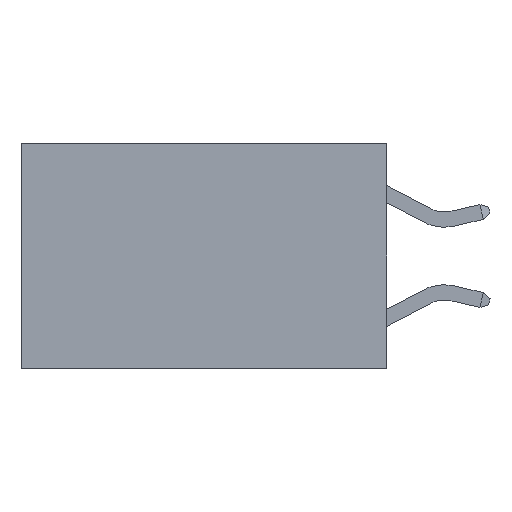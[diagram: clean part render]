
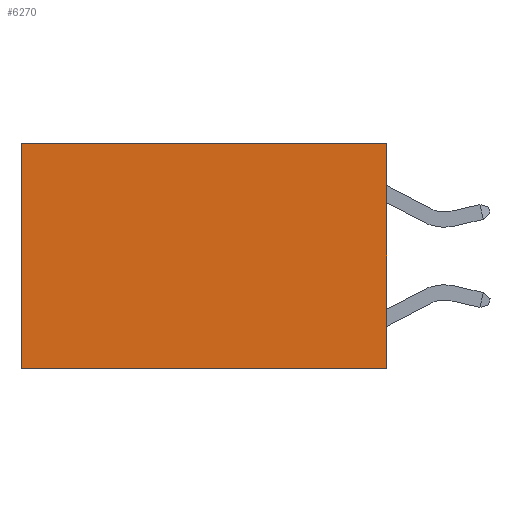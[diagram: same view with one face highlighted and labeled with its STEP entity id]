
A CAD part, left-side view. The second image highlights one B-rep face of the part: STEP entity #6270.
In plain terms, the highlighted planar face has unit normal (-1, 0, 0).
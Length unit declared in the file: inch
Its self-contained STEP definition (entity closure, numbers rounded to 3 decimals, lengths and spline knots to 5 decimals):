
#98 = ORIENTED_EDGE ( 'NONE', *, *, #858, .T. ) ;
#239 = VERTEX_POINT ( 'NONE', #744 ) ;
#382 = ORIENTED_EDGE ( 'NONE', *, *, #1693, .F. ) ;
#744 = CARTESIAN_POINT ( 'NONE',  ( 0.2625, 0.6, -0.37 ) ) ;
#858 = EDGE_CURVE ( 'NONE', #6455, #4580, #6442, .T. ) ;
#1083 = VERTEX_POINT ( 'NONE', #4020 ) ;
#1142 = EDGE_CURVE ( 'NONE', #6455, #1083, #1445, .T. ) ;
#1215 = AXIS2_PLACEMENT_3D ( 'NONE', #2213, #2033, #2023 ) ;
#1445 = LINE ( 'NONE', #8129, #4918 ) ;
#1579 = ORIENTED_EDGE ( 'NONE', *, *, #7103, .T. ) ;
#1693 = EDGE_CURVE ( 'NONE', #1083, #239, #5097, .T. ) ;
#2023 = DIRECTION ( 'NONE',  ( 0., 0., -1. ) ) ;
#2033 = DIRECTION ( 'NONE',  ( 1., 0., 0. ) ) ;
#2051 = PLANE ( 'NONE',  #1215 ) ;
#2061 = CARTESIAN_POINT ( 'NONE',  ( 0.2625, 0.6, 0. ) ) ;
#2064 = VECTOR ( 'NONE', #5233, 39.37008 ) ;
#2213 = CARTESIAN_POINT ( 'NONE',  ( 0.2625, 0., 0. ) ) ;
#3432 = DIRECTION ( 'NONE',  ( 0., 1., 0. ) ) ;
#3454 = EDGE_LOOP ( 'NONE', ( #1579, #382, #8194, #98 ) ) ;
#3459 = CARTESIAN_POINT ( 'NONE',  ( 0.2625, 0., -0.37 ) ) ;
#4020 = CARTESIAN_POINT ( 'NONE',  ( 0.2625, 0., -0.37 ) ) ;
#4046 = LINE ( 'NONE', #7254, #2064 ) ;
#4580 = VERTEX_POINT ( 'NONE', #2061 ) ;
#4609 = DIRECTION ( 'NONE',  ( 0., 0., -1. ) ) ;
#4611 = VECTOR ( 'NONE', #7429, 39.37008 ) ;
#4701 = VECTOR ( 'NONE', #3432, 39.37008 ) ;
#4918 = VECTOR ( 'NONE', #4609, 39.37008 ) ;
#5097 = LINE ( 'NONE', #3459, #4701 ) ;
#5233 = DIRECTION ( 'NONE',  ( 0., 0., -1. ) ) ;
#5687 = CARTESIAN_POINT ( 'NONE',  ( 0.2625, 0., 0. ) ) ;
#5986 = FACE_OUTER_BOUND ( 'NONE', #3454, .T. ) ;
#6270 = ADVANCED_FACE ( 'NONE', ( #5986 ), #2051, .F. ) ;
#6442 = LINE ( 'NONE', #7573, #4611 ) ;
#6455 = VERTEX_POINT ( 'NONE', #5687 ) ;
#7103 = EDGE_CURVE ( 'NONE', #4580, #239, #4046, .T. ) ;
#7254 = CARTESIAN_POINT ( 'NONE',  ( 0.2625, 0.6, 0. ) ) ;
#7429 = DIRECTION ( 'NONE',  ( 0., 1., 0. ) ) ;
#7573 = CARTESIAN_POINT ( 'NONE',  ( 0.2625, 0., 0. ) ) ;
#8129 = CARTESIAN_POINT ( 'NONE',  ( 0.2625, 0., 0. ) ) ;
#8194 = ORIENTED_EDGE ( 'NONE', *, *, #1142, .F. ) ;
